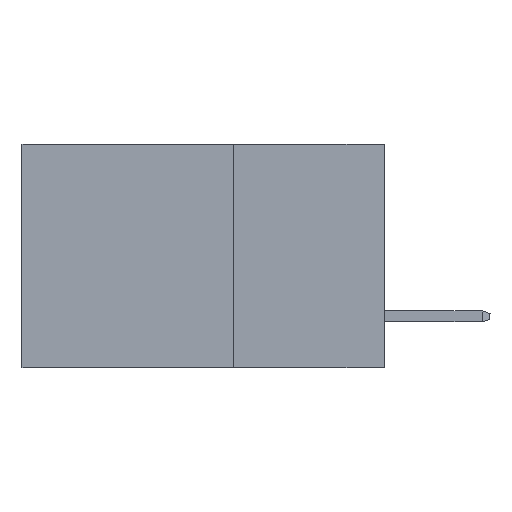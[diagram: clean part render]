
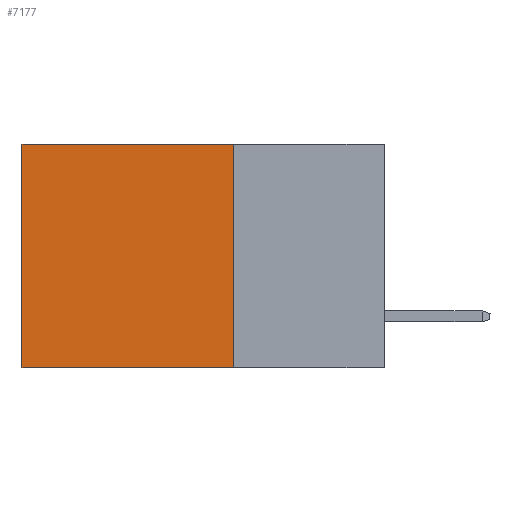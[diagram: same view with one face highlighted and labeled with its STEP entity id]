
A CAD part, left-side view. The second image highlights one B-rep face of the part: STEP entity #7177.
In plain terms, the highlighted planar face has unit normal (-1, 0, 0).
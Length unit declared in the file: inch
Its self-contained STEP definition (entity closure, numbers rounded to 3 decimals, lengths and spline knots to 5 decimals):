
#472 = DIRECTION ( 'NONE',  ( 0., 0., -1. ) ) ;
#538 = VERTEX_POINT ( 'NONE', #4184 ) ;
#580 = ORIENTED_EDGE ( 'NONE', *, *, #3198, .F. ) ;
#779 = ORIENTED_EDGE ( 'NONE', *, *, #4822, .T. ) ;
#1033 = FACE_OUTER_BOUND ( 'NONE', #2726, .T. ) ;
#1075 = CARTESIAN_POINT ( 'NONE',  ( 0.2615, 0.6, -0.37 ) ) ;
#1493 = LINE ( 'NONE', #10159, #9098 ) ;
#1827 = LINE ( 'NONE', #1075, #4228 ) ;
#2629 = PLANE ( 'NONE',  #6627 ) ;
#2726 = EDGE_LOOP ( 'NONE', ( #779, #9343, #580, #6467 ) ) ;
#3198 = EDGE_CURVE ( 'NONE', #7682, #6409, #8449, .T. ) ;
#4184 = CARTESIAN_POINT ( 'NONE',  ( 0.2615, 0.6, 0. ) ) ;
#4228 = VECTOR ( 'NONE', #4294, 39.37008 ) ;
#4294 = DIRECTION ( 'NONE',  ( 0., 0., -1. ) ) ;
#4655 = EDGE_CURVE ( 'NONE', #6409, #9971, #4776, .T. ) ;
#4667 = CARTESIAN_POINT ( 'NONE',  ( 0.2615, 0.25, 0. ) ) ;
#4776 = LINE ( 'NONE', #7187, #8743 ) ;
#4822 = EDGE_CURVE ( 'NONE', #538, #9971, #1827, .T. ) ;
#4949 = VECTOR ( 'NONE', #472, 39.37008 ) ;
#5082 = DIRECTION ( 'NONE',  ( 0., 0., -1. ) ) ;
#5107 = DIRECTION ( 'NONE',  ( 0., 1., 0. ) ) ;
#5656 = DIRECTION ( 'NONE',  ( 0., 1., 0. ) ) ;
#6409 = VERTEX_POINT ( 'NONE', #9085 ) ;
#6467 = ORIENTED_EDGE ( 'NONE', *, *, #6965, .T. ) ;
#6627 = AXIS2_PLACEMENT_3D ( 'NONE', #9781, #7371, #5082 ) ;
#6965 = EDGE_CURVE ( 'NONE', #7682, #538, #1493, .T. ) ;
#7177 = ADVANCED_FACE ( 'NONE', ( #1033 ), #2629, .F. ) ;
#7187 = CARTESIAN_POINT ( 'NONE',  ( 0.2615, 0.25, -0.37 ) ) ;
#7371 = DIRECTION ( 'NONE',  ( 1., 0., 0. ) ) ;
#7682 = VERTEX_POINT ( 'NONE', #4667 ) ;
#8208 = CARTESIAN_POINT ( 'NONE',  ( 0.2615, 0.6, -0.37 ) ) ;
#8449 = LINE ( 'NONE', #9848, #4949 ) ;
#8743 = VECTOR ( 'NONE', #5656, 39.37008 ) ;
#9085 = CARTESIAN_POINT ( 'NONE',  ( 0.2615, 0.25, -0.37 ) ) ;
#9098 = VECTOR ( 'NONE', #5107, 39.37008 ) ;
#9343 = ORIENTED_EDGE ( 'NONE', *, *, #4655, .F. ) ;
#9781 = CARTESIAN_POINT ( 'NONE',  ( 0.2615, 0.25, -0.37 ) ) ;
#9848 = CARTESIAN_POINT ( 'NONE',  ( 0.2615, 0.25, -0.37 ) ) ;
#9971 = VERTEX_POINT ( 'NONE', #8208 ) ;
#10159 = CARTESIAN_POINT ( 'NONE',  ( 0.2615, 0.25, 0. ) ) ;
